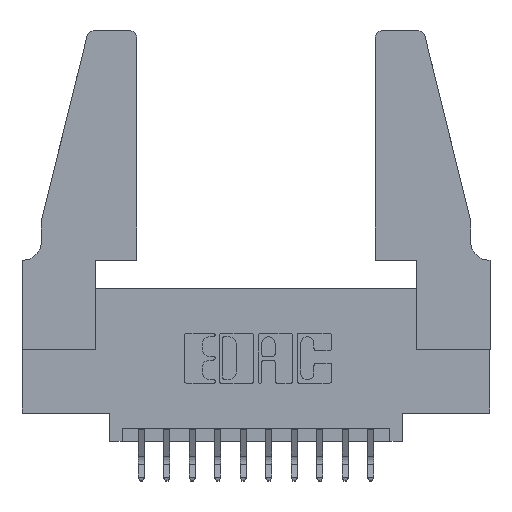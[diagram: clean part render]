
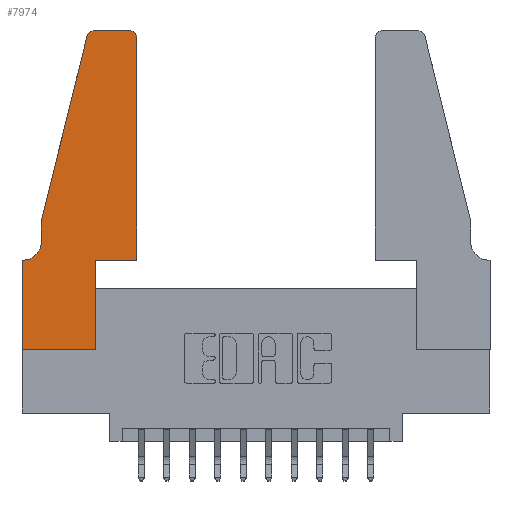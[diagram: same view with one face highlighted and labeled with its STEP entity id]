
A CAD part, top view. The second image highlights one B-rep face of the part: STEP entity #7974.
In plain terms, the highlighted planar face has unit normal (0, 0, 1).
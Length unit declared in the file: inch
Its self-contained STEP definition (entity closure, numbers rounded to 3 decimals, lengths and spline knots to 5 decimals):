
#138 = VERTEX_POINT ( 'NONE', #1375 ) ;
#149 = DIRECTION ( 'NONE',  ( 1., 0., 0. ) ) ;
#198 = CIRCLE ( 'NONE', #4901, 0.07 ) ;
#281 = LINE ( 'NONE', #11287, #8350 ) ;
#355 = VECTOR ( 'NONE', #2799, 39.37008 ) ;
#569 = CARTESIAN_POINT ( 'NONE',  ( 0.4505, 0.35, 0.37 ) ) ;
#1076 = CARTESIAN_POINT ( 'NONE',  ( 0.2865, 0., 0.37 ) ) ;
#1329 = CARTESIAN_POINT ( 'NONE',  ( 0.4505, 1.22, 0.37 ) ) ;
#1332 = DIRECTION ( 'NONE',  ( 0., 0., -1. ) ) ;
#1360 = EDGE_CURVE ( 'NONE', #9697, #7112, #6553, .T. ) ;
#1375 = CARTESIAN_POINT ( 'NONE',  ( 0.284, 1.25, 0.37 ) ) ;
#1859 = ORIENTED_EDGE ( 'NONE', *, *, #8089, .T. ) ;
#1963 = CARTESIAN_POINT ( 'NONE',  ( 0., 0., 0.37 ) ) ;
#2336 = DIRECTION ( 'NONE',  ( 0., 0., 1. ) ) ;
#2626 = ORIENTED_EDGE ( 'NONE', *, *, #6322, .T. ) ;
#2696 = CARTESIAN_POINT ( 'NONE',  ( 0.2865, 0.35, 0.37 ) ) ;
#2799 = DIRECTION ( 'NONE',  ( 1., 0., 0. ) ) ;
#2907 = VECTOR ( 'NONE', #4371, 39.37008 ) ;
#2929 = CARTESIAN_POINT ( 'NONE',  ( 0.4205, 1.25, 0.37 ) ) ;
#3074 = CIRCLE ( 'NONE', #3143, 0.03 ) ;
#3143 = AXIS2_PLACEMENT_3D ( 'NONE', #9124, #2336, #10232 ) ;
#3306 = DIRECTION ( 'NONE',  ( 0., 1., 0. ) ) ;
#3477 = LINE ( 'NONE', #13950, #355 ) ;
#3592 = VERTEX_POINT ( 'NONE', #4567 ) ;
#3673 = ORIENTED_EDGE ( 'NONE', *, *, #7893, .T. ) ;
#3758 = VECTOR ( 'NONE', #3306, 39.37008 ) ;
#4001 = EDGE_CURVE ( 'NONE', #7112, #4980, #10385, .T. ) ;
#4371 = DIRECTION ( 'NONE',  ( -1., 0., 0. ) ) ;
#4567 = CARTESIAN_POINT ( 'NONE',  ( 0.0755, 0.5, 0.37 ) ) ;
#4627 = DIRECTION ( 'NONE',  ( -0.239, -0.971, 0. ) ) ;
#4682 = LINE ( 'NONE', #11600, #12921 ) ;
#4851 = VERTEX_POINT ( 'NONE', #1076 ) ;
#4901 = AXIS2_PLACEMENT_3D ( 'NONE', #8152, #1332, #9287 ) ;
#4980 = VERTEX_POINT ( 'NONE', #1329 ) ;
#4992 = VECTOR ( 'NONE', #4627, 39.37008 ) ;
#5253 = DIRECTION ( 'NONE',  ( -1., 0., 0. ) ) ;
#5577 = CARTESIAN_POINT ( 'NONE',  ( 0.2865, 0.35, 0.37 ) ) ;
#5588 = ORIENTED_EDGE ( 'NONE', *, *, #4001, .T. ) ;
#5665 = EDGE_CURVE ( 'NONE', #7231, #4851, #3477, .T. ) ;
#5678 = ORIENTED_EDGE ( 'NONE', *, *, #11373, .T. ) ;
#5719 = DIRECTION ( 'NONE',  ( 0., -1., 0. ) ) ;
#5738 = PLANE ( 'NONE',  #8009 ) ;
#5790 = EDGE_LOOP ( 'NONE', ( #7419, #1859, #7564, #2626, #11482, #10173, #12850, #6451, #3673, #8188, #5588, #5678 ) ) ;
#6035 = DIRECTION ( 'NONE',  ( 0., -1., 0. ) ) ;
#6322 = EDGE_CURVE ( 'NONE', #3592, #6361, #4682, .T. ) ;
#6361 = VERTEX_POINT ( 'NONE', #7205 ) ;
#6451 = ORIENTED_EDGE ( 'NONE', *, *, #5665, .T. ) ;
#6553 = LINE ( 'NONE', #10684, #12131 ) ;
#6875 = DIRECTION ( 'NONE',  ( 1., 0., 0. ) ) ;
#7068 = DIRECTION ( 'NONE',  ( 0., 0., 1. ) ) ;
#7112 = VERTEX_POINT ( 'NONE', #569 ) ;
#7205 = CARTESIAN_POINT ( 'NONE',  ( 0.0755, 0.42, 0.37 ) ) ;
#7231 = VERTEX_POINT ( 'NONE', #1963 ) ;
#7291 = CIRCLE ( 'NONE', #10989, 0.03 ) ;
#7419 = ORIENTED_EDGE ( 'NONE', *, *, #11241, .T. ) ;
#7564 = ORIENTED_EDGE ( 'NONE', *, *, #12296, .T. ) ;
#7598 = VERTEX_POINT ( 'NONE', #9388 ) ;
#7893 = EDGE_CURVE ( 'NONE', #4851, #9697, #10106, .T. ) ;
#7974 = ADVANCED_FACE ( 'NONE', ( #9057 ), #5738, .T. ) ;
#8009 = AXIS2_PLACEMENT_3D ( 'NONE', #10198, #13536, #6875 ) ;
#8089 = EDGE_CURVE ( 'NONE', #138, #11343, #7291, .T. ) ;
#8152 = CARTESIAN_POINT ( 'NONE',  ( 0.0055, 0.42, 0.37 ) ) ;
#8188 = ORIENTED_EDGE ( 'NONE', *, *, #1360, .T. ) ;
#8350 = VECTOR ( 'NONE', #5719, 39.37008 ) ;
#8965 = EDGE_CURVE ( 'NONE', #6361, #7598, #198, .T. ) ;
#9048 = LINE ( 'NONE', #9696, #11652 ) ;
#9057 = FACE_OUTER_BOUND ( 'NONE', #5790, .T. ) ;
#9074 = CARTESIAN_POINT ( 'NONE',  ( 0.25487, 1.22718, 0.37 ) ) ;
#9124 = CARTESIAN_POINT ( 'NONE',  ( 0.4205, 1.22, 0.37 ) ) ;
#9287 = DIRECTION ( 'NONE',  ( -1., 0., 0. ) ) ;
#9388 = CARTESIAN_POINT ( 'NONE',  ( 0.0055, 0.35, 0.37 ) ) ;
#9696 = CARTESIAN_POINT ( 'NONE',  ( 0.0755, 0.35, 0.37 ) ) ;
#9697 = VERTEX_POINT ( 'NONE', #2696 ) ;
#9848 = DIRECTION ( 'NONE',  ( 0., 1., 0. ) ) ;
#10046 = VECTOR ( 'NONE', #9848, 39.37008 ) ;
#10106 = LINE ( 'NONE', #5577, #3758 ) ;
#10173 = ORIENTED_EDGE ( 'NONE', *, *, #13323, .T. ) ;
#10198 = CARTESIAN_POINT ( 'NONE',  ( 0., 0.35, 0.37 ) ) ;
#10232 = DIRECTION ( 'NONE',  ( 1., 0., 0. ) ) ;
#10267 = LINE ( 'NONE', #11349, #4992 ) ;
#10385 = LINE ( 'NONE', #14231, #10046 ) ;
#10512 = DIRECTION ( 'NONE',  ( 1., 0., 0. ) ) ;
#10684 = CARTESIAN_POINT ( 'NONE',  ( 0.4505, 0.35, 0.37 ) ) ;
#10989 = AXIS2_PLACEMENT_3D ( 'NONE', #13719, #7068, #149 ) ;
#11095 = CARTESIAN_POINT ( 'NONE',  ( 0.2605, 1.25, 0.37 ) ) ;
#11241 = EDGE_CURVE ( 'NONE', #13304, #138, #13431, .T. ) ;
#11287 = CARTESIAN_POINT ( 'NONE',  ( 0., 0., 0.37 ) ) ;
#11343 = VERTEX_POINT ( 'NONE', #9074 ) ;
#11349 = CARTESIAN_POINT ( 'NONE',  ( 0.0755, 0.5, 0.37 ) ) ;
#11373 = EDGE_CURVE ( 'NONE', #4980, #13304, #3074, .T. ) ;
#11482 = ORIENTED_EDGE ( 'NONE', *, *, #8965, .T. ) ;
#11600 = CARTESIAN_POINT ( 'NONE',  ( 0.0755, 0.5, 0.37 ) ) ;
#11652 = VECTOR ( 'NONE', #5253, 39.37008 ) ;
#12131 = VECTOR ( 'NONE', #10512, 39.37008 ) ;
#12296 = EDGE_CURVE ( 'NONE', #11343, #3592, #10267, .T. ) ;
#12782 = VERTEX_POINT ( 'NONE', #14344 ) ;
#12850 = ORIENTED_EDGE ( 'NONE', *, *, #12928, .T. ) ;
#12921 = VECTOR ( 'NONE', #6035, 39.37008 ) ;
#12928 = EDGE_CURVE ( 'NONE', #12782, #7231, #281, .T. ) ;
#13304 = VERTEX_POINT ( 'NONE', #2929 ) ;
#13323 = EDGE_CURVE ( 'NONE', #7598, #12782, #9048, .T. ) ;
#13431 = LINE ( 'NONE', #11095, #2907 ) ;
#13536 = DIRECTION ( 'NONE',  ( 0., 0., 1. ) ) ;
#13719 = CARTESIAN_POINT ( 'NONE',  ( 0.284, 1.22, 0.37 ) ) ;
#13950 = CARTESIAN_POINT ( 'NONE',  ( 0., 0., 0.37 ) ) ;
#14231 = CARTESIAN_POINT ( 'NONE',  ( 0.4505, 0.35, 0.37 ) ) ;
#14344 = CARTESIAN_POINT ( 'NONE',  ( 0., 0.35, 0.37 ) ) ;
